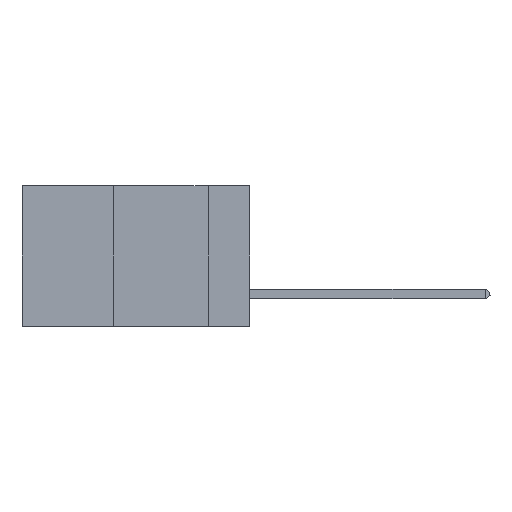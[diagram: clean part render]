
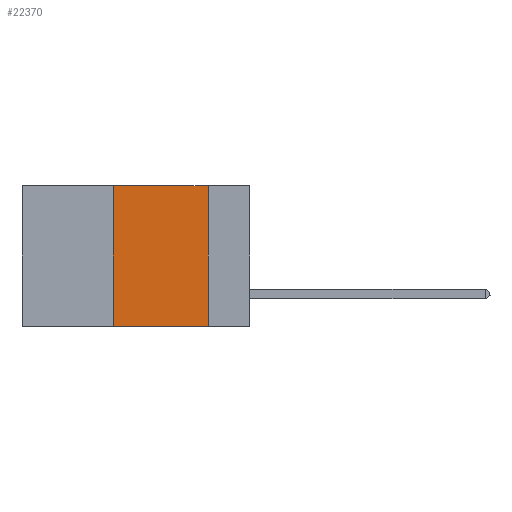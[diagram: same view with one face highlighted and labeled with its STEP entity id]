
A CAD part, left-side view. The second image highlights one B-rep face of the part: STEP entity #22370.
In plain terms, the highlighted planar face has unit normal (-1, 0, 0).
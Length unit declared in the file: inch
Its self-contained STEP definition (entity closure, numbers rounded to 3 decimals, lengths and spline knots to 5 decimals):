
#1200 = CARTESIAN_POINT ( 'NONE',  ( 0., 0.36, -0.37 ) ) ;
#2109 = CARTESIAN_POINT ( 'NONE',  ( 0., 0.6, 0. ) ) ;
#2227 = CARTESIAN_POINT ( 'NONE',  ( 0., 0.36, 0. ) ) ;
#4182 = CARTESIAN_POINT ( 'NONE',  ( 0., 0.36, 0. ) ) ;
#9594 = CARTESIAN_POINT ( 'NONE',  ( 0., 0.11, -0.37 ) ) ;
#11410 = ORIENTED_EDGE ( 'NONE', *, *, #35410, .F. ) ;
#11576 = CARTESIAN_POINT ( 'NONE',  ( 0., 0.6, -0.37 ) ) ;
#11617 = DIRECTION ( 'NONE',  ( 0., 0., 1. ) ) ;
#12582 = EDGE_CURVE ( 'NONE', #13682, #13952, #17011, .T. ) ;
#12955 = AXIS2_PLACEMENT_3D ( 'NONE', #2109, #22887, #20424 ) ;
#13682 = VERTEX_POINT ( 'NONE', #22085 ) ;
#13952 = VERTEX_POINT ( 'NONE', #9594 ) ;
#16986 = FACE_OUTER_BOUND ( 'NONE', #36799, .T. ) ;
#17011 = LINE ( 'NONE', #29391, #19904 ) ;
#17511 = LINE ( 'NONE', #2227, #36355 ) ;
#18639 = VERTEX_POINT ( 'NONE', #1200 ) ;
#19904 = VECTOR ( 'NONE', #29984, 39.37008 ) ;
#19991 = EDGE_CURVE ( 'NONE', #18639, #13952, #40037, .T. ) ;
#20424 = DIRECTION ( 'NONE',  ( 0., 0., -1. ) ) ;
#20536 = LINE ( 'NONE', #23408, #33095 ) ;
#22085 = CARTESIAN_POINT ( 'NONE',  ( 0., 0.11, 0. ) ) ;
#22370 = ADVANCED_FACE ( 'NONE', ( #16986 ), #35889, .F. ) ;
#22887 = DIRECTION ( 'NONE',  ( 1., 0., 0. ) ) ;
#23233 = ORIENTED_EDGE ( 'NONE', *, *, #19991, .T. ) ;
#23408 = CARTESIAN_POINT ( 'NONE',  ( 0., 0.6, 0. ) ) ;
#23964 = DIRECTION ( 'NONE',  ( 0., -1., 0. ) ) ;
#24502 = VECTOR ( 'NONE', #23964, 39.37008 ) ;
#26155 = ORIENTED_EDGE ( 'NONE', *, *, #12582, .F. ) ;
#28574 = EDGE_CURVE ( 'NONE', #29220, #13682, #20536, .T. ) ;
#29220 = VERTEX_POINT ( 'NONE', #4182 ) ;
#29391 = CARTESIAN_POINT ( 'NONE',  ( 0., 0.11, 0. ) ) ;
#29984 = DIRECTION ( 'NONE',  ( 0., 0., -1. ) ) ;
#31345 = ORIENTED_EDGE ( 'NONE', *, *, #28574, .F. ) ;
#33095 = VECTOR ( 'NONE', #39678, 39.37008 ) ;
#35410 = EDGE_CURVE ( 'NONE', #18639, #29220, #17511, .T. ) ;
#35889 = PLANE ( 'NONE',  #12955 ) ;
#36355 = VECTOR ( 'NONE', #11617, 39.37008 ) ;
#36799 = EDGE_LOOP ( 'NONE', ( #26155, #31345, #11410, #23233 ) ) ;
#39678 = DIRECTION ( 'NONE',  ( 0., -1., 0. ) ) ;
#40037 = LINE ( 'NONE', #11576, #24502 ) ;
